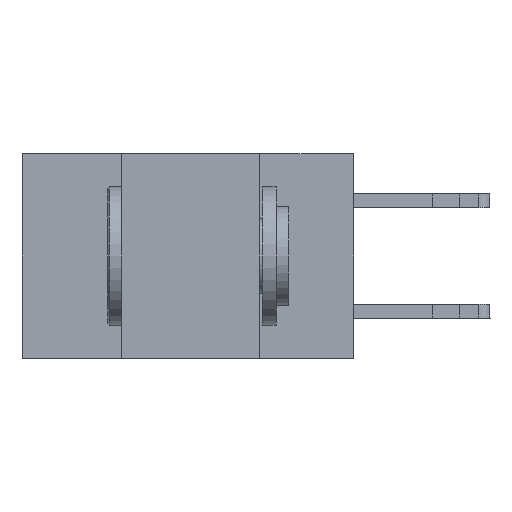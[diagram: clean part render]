
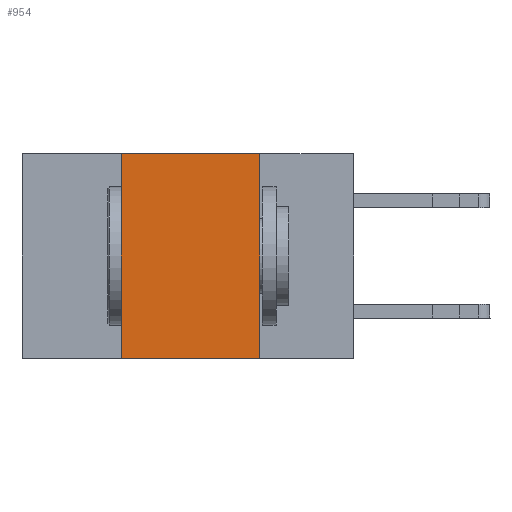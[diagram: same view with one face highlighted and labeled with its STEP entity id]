
A CAD part, left-side view. The second image highlights one B-rep face of the part: STEP entity #954.
In plain terms, the highlighted planar face has unit normal (-1, 0, 0).
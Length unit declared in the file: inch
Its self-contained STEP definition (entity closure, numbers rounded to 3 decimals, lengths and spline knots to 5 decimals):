
#379 = CARTESIAN_POINT ( 'NONE',  ( 0., 0.17, -0.37 ) ) ;
#405 = VERTEX_POINT ( 'NONE', #19130 ) ;
#695 = ORIENTED_EDGE ( 'NONE', *, *, #4774, .T. ) ;
#954 = ADVANCED_FACE ( 'NONE', ( #19102 ), #6746, .F. ) ;
#1150 = VECTOR ( 'NONE', #4659, 39.37008 ) ;
#1910 = VECTOR ( 'NONE', #6361, 39.37008 ) ;
#2380 = AXIS2_PLACEMENT_3D ( 'NONE', #6723, #6665, #6642 ) ;
#2507 = ORIENTED_EDGE ( 'NONE', *, *, #18366, .F. ) ;
#3337 = EDGE_CURVE ( 'NONE', #13125, #405, #15264, .T. ) ;
#3769 = ORIENTED_EDGE ( 'NONE', *, *, #3337, .F. ) ;
#4659 = DIRECTION ( 'NONE',  ( 0., -1., 0. ) ) ;
#4681 = CARTESIAN_POINT ( 'NONE',  ( 0., 0.6, 0. ) ) ;
#4774 = EDGE_CURVE ( 'NONE', #5116, #7606, #17197, .T. ) ;
#5116 = VERTEX_POINT ( 'NONE', #22389 ) ;
#6361 = DIRECTION ( 'NONE',  ( 0., -1., 0. ) ) ;
#6642 = DIRECTION ( 'NONE',  ( 0., 0., -1. ) ) ;
#6665 = DIRECTION ( 'NONE',  ( 1., 0., 0. ) ) ;
#6723 = CARTESIAN_POINT ( 'NONE',  ( 0., 0.6, 0. ) ) ;
#6746 = PLANE ( 'NONE',  #2380 ) ;
#7606 = VERTEX_POINT ( 'NONE', #379 ) ;
#7676 = CARTESIAN_POINT ( 'NONE',  ( 0., 0.17, 0. ) ) ;
#9296 = EDGE_LOOP ( 'NONE', ( #14986, #3769, #2507, #695 ) ) ;
#9547 = DIRECTION ( 'NONE',  ( 0., 0., -1. ) ) ;
#12676 = CARTESIAN_POINT ( 'NONE',  ( 0., 0.42, 0. ) ) ;
#13125 = VERTEX_POINT ( 'NONE', #16832 ) ;
#13949 = VECTOR ( 'NONE', #14471, 39.37008 ) ;
#14471 = DIRECTION ( 'NONE',  ( 0., 0., 1. ) ) ;
#14986 = ORIENTED_EDGE ( 'NONE', *, *, #23508, .F. ) ;
#15046 = LINE ( 'NONE', #12676, #13949 ) ;
#15264 = LINE ( 'NONE', #4681, #1150 ) ;
#16428 = CARTESIAN_POINT ( 'NONE',  ( 0., 0.6, -0.37 ) ) ;
#16548 = VECTOR ( 'NONE', #9547, 39.37008 ) ;
#16832 = CARTESIAN_POINT ( 'NONE',  ( 0., 0.42, 0. ) ) ;
#17197 = LINE ( 'NONE', #16428, #1910 ) ;
#18366 = EDGE_CURVE ( 'NONE', #5116, #13125, #15046, .T. ) ;
#19102 = FACE_OUTER_BOUND ( 'NONE', #9296, .T. ) ;
#19130 = CARTESIAN_POINT ( 'NONE',  ( 0., 0.17, 0. ) ) ;
#21374 = LINE ( 'NONE', #7676, #16548 ) ;
#22389 = CARTESIAN_POINT ( 'NONE',  ( 0., 0.42, -0.37 ) ) ;
#23508 = EDGE_CURVE ( 'NONE', #405, #7606, #21374, .T. ) ;
